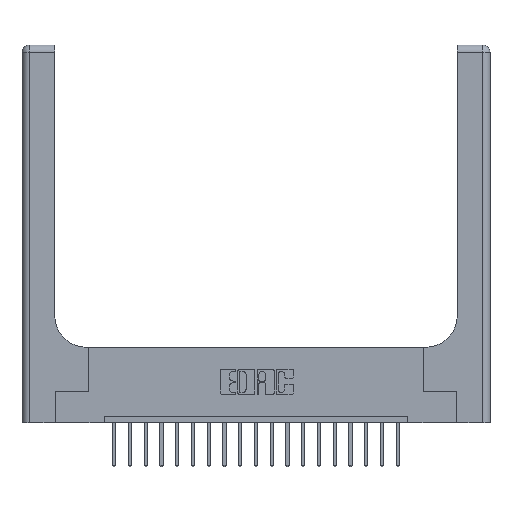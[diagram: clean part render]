
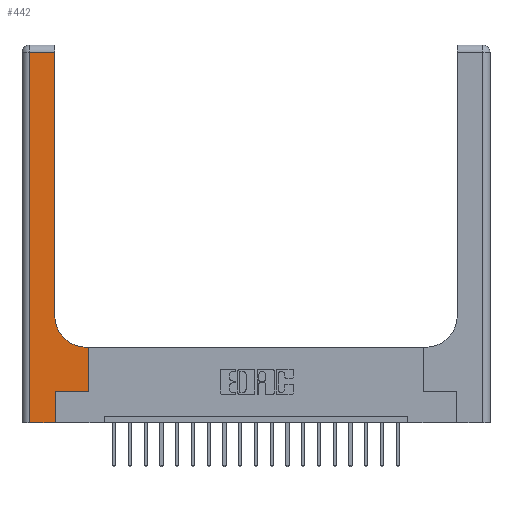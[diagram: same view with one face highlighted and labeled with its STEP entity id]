
A CAD part, top view. The second image highlights one B-rep face of the part: STEP entity #442.
In plain terms, the highlighted planar face has unit normal (0, 0, 1).
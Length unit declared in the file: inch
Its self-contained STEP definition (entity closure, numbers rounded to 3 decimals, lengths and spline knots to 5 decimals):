
#442 = ADVANCED_FACE ( 'NONE', ( #19937 ), #13839, .F. ) ;
#647 = VERTEX_POINT ( 'NONE', #5418 ) ;
#924 = EDGE_CURVE ( 'NONE', #1813, #2011, #5163, .T. ) ;
#1023 = ORIENTED_EDGE ( 'NONE', *, *, #3928, .T. ) ;
#1586 = CARTESIAN_POINT ( 'NONE',  ( 0.26, 2.94, 0.37 ) ) ;
#1648 = VECTOR ( 'NONE', #16090, 39.37008 ) ;
#1813 = VERTEX_POINT ( 'NONE', #4425 ) ;
#1975 = EDGE_CURVE ( 'NONE', #6071, #19749, #18714, .T. ) ;
#2011 = VERTEX_POINT ( 'NONE', #9407 ) ;
#3903 = CARTESIAN_POINT ( 'NONE',  ( 0.528, 0.6, 0.37 ) ) ;
#3928 = EDGE_CURVE ( 'NONE', #15868, #6071, #16807, .T. ) ;
#4122 = ORIENTED_EDGE ( 'NONE', *, *, #924, .T. ) ;
#4284 = VECTOR ( 'NONE', #11440, 39.37008 ) ;
#4292 = CARTESIAN_POINT ( 'NONE',  ( 0., 3., 0.37 ) ) ;
#4425 = CARTESIAN_POINT ( 'NONE',  ( 0.265, 0.25, 0.37 ) ) ;
#4734 = CARTESIAN_POINT ( 'NONE',  ( 0., 0., 0.37 ) ) ;
#4931 = DIRECTION ( 'NONE',  ( 0., 0., -1. ) ) ;
#5163 = LINE ( 'NONE', #11603, #14378 ) ;
#5359 = CARTESIAN_POINT ( 'NONE',  ( 0., 2.94, 0.37 ) ) ;
#5407 = ORIENTED_EDGE ( 'NONE', *, *, #15343, .T. ) ;
#5418 = CARTESIAN_POINT ( 'NONE',  ( 0.51, 0.6, 0.37 ) ) ;
#5528 = ORIENTED_EDGE ( 'NONE', *, *, #7248, .T. ) ;
#5566 = ORIENTED_EDGE ( 'NONE', *, *, #14153, .T. ) ;
#6071 = VERTEX_POINT ( 'NONE', #6551 ) ;
#6551 = CARTESIAN_POINT ( 'NONE',  ( 0.06, 0., 0.37 ) ) ;
#7232 = VECTOR ( 'NONE', #15722, 39.37008 ) ;
#7248 = EDGE_CURVE ( 'NONE', #19927, #15868, #14891, .T. ) ;
#8149 = CARTESIAN_POINT ( 'NONE',  ( 0.51, 0.85, 0.37 ) ) ;
#8917 = VECTOR ( 'NONE', #11690, 39.37008 ) ;
#9407 = CARTESIAN_POINT ( 'NONE',  ( 0.528, 0.25, 0.37 ) ) ;
#9794 = CARTESIAN_POINT ( 'NONE',  ( 0.26, 3., 0.37 ) ) ;
#10359 = CARTESIAN_POINT ( 'NONE',  ( 0.528, 0.25, 0.37 ) ) ;
#10916 = EDGE_CURVE ( 'NONE', #11914, #19927, #19514, .T. ) ;
#11240 = CARTESIAN_POINT ( 'NONE',  ( 0.26, 0.6, 0.37 ) ) ;
#11270 = DIRECTION ( 'NONE',  ( 1., 0., 0. ) ) ;
#11350 = CARTESIAN_POINT ( 'NONE',  ( 0.26, 0.85, 0.37 ) ) ;
#11436 = ORIENTED_EDGE ( 'NONE', *, *, #10916, .T. ) ;
#11440 = DIRECTION ( 'NONE',  ( -1., 0., 0. ) ) ;
#11603 = CARTESIAN_POINT ( 'NONE',  ( 0.265, 0.25, 0.37 ) ) ;
#11690 = DIRECTION ( 'NONE',  ( -1., 0., 0. ) ) ;
#11827 = CARTESIAN_POINT ( 'NONE',  ( 0.06, 2.94, 0.37 ) ) ;
#11914 = VERTEX_POINT ( 'NONE', #11350 ) ;
#12048 = ORIENTED_EDGE ( 'NONE', *, *, #1975, .T. ) ;
#12102 = ORIENTED_EDGE ( 'NONE', *, *, #14969, .T. ) ;
#12147 = EDGE_LOOP ( 'NONE', ( #11436, #5528, #1023, #12048, #5407, #4122, #14982, #5566, #12102 ) ) ;
#12895 = LINE ( 'NONE', #14544, #1648 ) ;
#13633 = DIRECTION ( 'NONE',  ( 0., 0., -1. ) ) ;
#13839 = PLANE ( 'NONE',  #14024 ) ;
#13972 = VECTOR ( 'NONE', #16867, 39.37008 ) ;
#14024 = AXIS2_PLACEMENT_3D ( 'NONE', #4292, #13633, #20147 ) ;
#14153 = EDGE_CURVE ( 'NONE', #18759, #647, #19091, .T. ) ;
#14378 = VECTOR ( 'NONE', #17319, 39.37008 ) ;
#14544 = CARTESIAN_POINT ( 'NONE',  ( 0.265, 0., 0.37 ) ) ;
#14891 = LINE ( 'NONE', #5359, #8917 ) ;
#14969 = EDGE_CURVE ( 'NONE', #647, #11914, #20521, .T. ) ;
#14982 = ORIENTED_EDGE ( 'NONE', *, *, #17039, .T. ) ;
#15044 = VECTOR ( 'NONE', #18058, 39.37008 ) ;
#15343 = EDGE_CURVE ( 'NONE', #19749, #1813, #12895, .T. ) ;
#15366 = CARTESIAN_POINT ( 'NONE',  ( 0.06, 3., 0.37 ) ) ;
#15565 = AXIS2_PLACEMENT_3D ( 'NONE', #8149, #4931, #11270 ) ;
#15722 = DIRECTION ( 'NONE',  ( 1., 0., 0. ) ) ;
#15868 = VERTEX_POINT ( 'NONE', #11827 ) ;
#16090 = DIRECTION ( 'NONE',  ( 0., 1., 0. ) ) ;
#16194 = DIRECTION ( 'NONE',  ( 0., 1., 0. ) ) ;
#16807 = LINE ( 'NONE', #15366, #15044 ) ;
#16867 = DIRECTION ( 'NONE',  ( 0., 1., 0. ) ) ;
#17039 = EDGE_CURVE ( 'NONE', #2011, #18759, #18216, .T. ) ;
#17319 = DIRECTION ( 'NONE',  ( 1., 0., 0. ) ) ;
#18058 = DIRECTION ( 'NONE',  ( 0., -1., 0. ) ) ;
#18130 = VECTOR ( 'NONE', #16194, 39.37008 ) ;
#18216 = LINE ( 'NONE', #10359, #13972 ) ;
#18714 = LINE ( 'NONE', #4734, #7232 ) ;
#18759 = VERTEX_POINT ( 'NONE', #3903 ) ;
#19091 = LINE ( 'NONE', #11240, #4284 ) ;
#19514 = LINE ( 'NONE', #9794, #18130 ) ;
#19553 = CARTESIAN_POINT ( 'NONE',  ( 0.265, 0., 0.37 ) ) ;
#19749 = VERTEX_POINT ( 'NONE', #19553 ) ;
#19927 = VERTEX_POINT ( 'NONE', #1586 ) ;
#19937 = FACE_OUTER_BOUND ( 'NONE', #12147, .T. ) ;
#20147 = DIRECTION ( 'NONE',  ( -1., 0., 0. ) ) ;
#20521 = CIRCLE ( 'NONE', #15565, 0.25 ) ;
